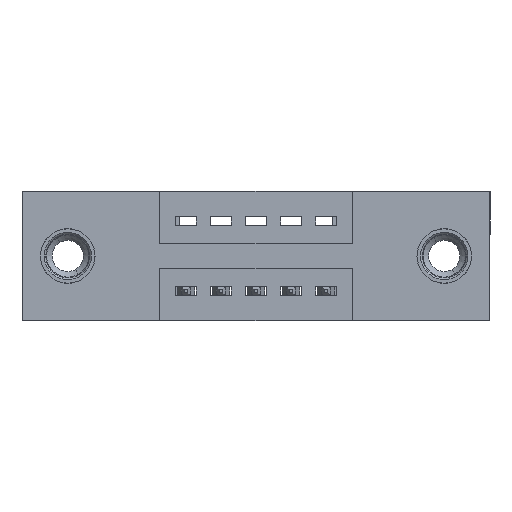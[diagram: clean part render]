
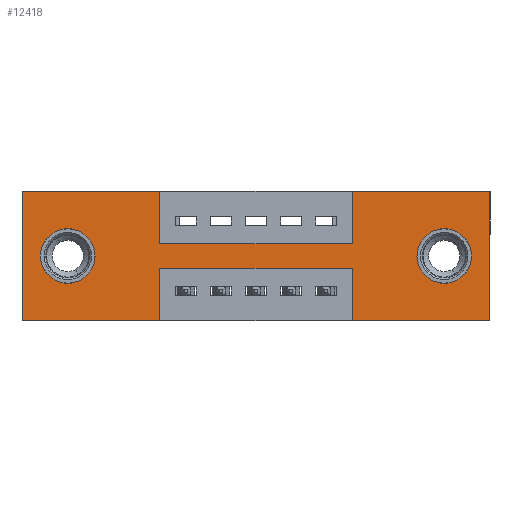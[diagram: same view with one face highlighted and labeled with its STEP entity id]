
A CAD part, front view. The second image highlights one B-rep face of the part: STEP entity #12418.
In plain terms, the highlighted planar face has unit normal (0, -1, 0).
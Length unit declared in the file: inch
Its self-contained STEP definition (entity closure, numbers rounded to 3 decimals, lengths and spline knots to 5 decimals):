
#65 = VERTEX_POINT ( 'NONE', #7563 ) ;
#151 = ORIENTED_EDGE ( 'NONE', *, *, #4716, .T. ) ;
#329 = DIRECTION ( 'NONE',  ( 0., 0., -1. ) ) ;
#368 = CARTESIAN_POINT ( 'NONE',  ( 0.13, 0., -0.263 ) ) ;
#464 = VECTOR ( 'NONE', #4039, 39.37008 ) ;
#468 = CARTESIAN_POINT ( 'NONE',  ( 0.3925, 0., -0.15 ) ) ;
#553 = AXIS2_PLACEMENT_3D ( 'NONE', #3110, #9493, #3149 ) ;
#770 = CARTESIAN_POINT ( 'NONE',  ( 1.205, 0., -0.185 ) ) ;
#801 = EDGE_CURVE ( 'NONE', #4588, #1624, #7181, .T. ) ;
#864 = LINE ( 'NONE', #12843, #6256 ) ;
#886 = CARTESIAN_POINT ( 'NONE',  ( 0.3925, 0., -0.37 ) ) ;
#897 = CARTESIAN_POINT ( 'NONE',  ( 0., 0., 0. ) ) ;
#1058 = EDGE_CURVE ( 'NONE', #5601, #1736, #4562, .T. ) ;
#1061 = VECTOR ( 'NONE', #6084, 39.37008 ) ;
#1085 = CARTESIAN_POINT ( 'NONE',  ( 1.335, 0., -0.37 ) ) ;
#1220 = LINE ( 'NONE', #897, #1061 ) ;
#1275 = VERTEX_POINT ( 'NONE', #5550 ) ;
#1297 = EDGE_CURVE ( 'NONE', #10303, #12620, #2593, .T. ) ;
#1338 = DIRECTION ( 'NONE',  ( 0., 0., 1. ) ) ;
#1624 = VERTEX_POINT ( 'NONE', #10181 ) ;
#1698 = DIRECTION ( 'NONE',  ( 1., 0., 0. ) ) ;
#1736 = VERTEX_POINT ( 'NONE', #12914 ) ;
#1891 = CARTESIAN_POINT ( 'NONE',  ( 0.9425, 0., -0.37 ) ) ;
#1957 = DIRECTION ( 'NONE',  ( -1., 0., 0. ) ) ;
#2049 = VERTEX_POINT ( 'NONE', #1085 ) ;
#2059 = ORIENTED_EDGE ( 'NONE', *, *, #7892, .F. ) ;
#2263 = DIRECTION ( 'NONE',  ( 1., 0., 0. ) ) ;
#2427 = CARTESIAN_POINT ( 'NONE',  ( 0., 0., 0. ) ) ;
#2509 = CIRCLE ( 'NONE', #6587, 0.078 ) ;
#2593 = CIRCLE ( 'NONE', #12894, 0.078 ) ;
#2631 = AXIS2_PLACEMENT_3D ( 'NONE', #3079, #10369, #8217 ) ;
#2674 = CARTESIAN_POINT ( 'NONE',  ( 0.3925, 0., -0.15 ) ) ;
#2744 = ORIENTED_EDGE ( 'NONE', *, *, #1058, .F. ) ;
#2824 = LINE ( 'NONE', #6087, #10468 ) ;
#2973 = EDGE_CURVE ( 'NONE', #9073, #12491, #11441, .T. ) ;
#3069 = CARTESIAN_POINT ( 'NONE',  ( 0.3925, 0., 0. ) ) ;
#3079 = CARTESIAN_POINT ( 'NONE',  ( 0.13, 0., -0.185 ) ) ;
#3110 = CARTESIAN_POINT ( 'NONE',  ( 0., 0., -0.37 ) ) ;
#3149 = DIRECTION ( 'NONE',  ( 0., 0., -1. ) ) ;
#3152 = EDGE_LOOP ( 'NONE', ( #11477, #5903 ) ) ;
#3196 = PLANE ( 'NONE',  #553 ) ;
#3593 = VERTEX_POINT ( 'NONE', #12208 ) ;
#3740 = CARTESIAN_POINT ( 'NONE',  ( 1.205, 0., -0.185 ) ) ;
#4039 = DIRECTION ( 'NONE',  ( -1., 0., 0. ) ) ;
#4060 = VECTOR ( 'NONE', #1338, 39.37008 ) ;
#4089 = ORIENTED_EDGE ( 'NONE', *, *, #2973, .F. ) ;
#4096 = VECTOR ( 'NONE', #6308, 39.37008 ) ;
#4217 = CARTESIAN_POINT ( 'NONE',  ( 0.3925, 0., 0. ) ) ;
#4244 = ORIENTED_EDGE ( 'NONE', *, *, #5753, .F. ) ;
#4419 = CARTESIAN_POINT ( 'NONE',  ( 0.3925, 0., -0.22 ) ) ;
#4469 = DIRECTION ( 'NONE',  ( -1., 0., 0. ) ) ;
#4562 = LINE ( 'NONE', #11212, #464 ) ;
#4588 = VERTEX_POINT ( 'NONE', #468 ) ;
#4716 = EDGE_CURVE ( 'NONE', #12620, #10303, #12542, .T. ) ;
#4994 = VECTOR ( 'NONE', #1957, 39.37008 ) ;
#5079 = VERTEX_POINT ( 'NONE', #5829 ) ;
#5218 = CARTESIAN_POINT ( 'NONE',  ( 0.9425, 0., -0.22 ) ) ;
#5248 = CARTESIAN_POINT ( 'NONE',  ( 0.13, 0., -0.107 ) ) ;
#5309 = CARTESIAN_POINT ( 'NONE',  ( 0.9425, 0., -0.37 ) ) ;
#5371 = FACE_OUTER_BOUND ( 'NONE', #10951, .T. ) ;
#5502 = LINE ( 'NONE', #2427, #4060 ) ;
#5550 = CARTESIAN_POINT ( 'NONE',  ( 1.205, 0., -0.107 ) ) ;
#5601 = VERTEX_POINT ( 'NONE', #886 ) ;
#5628 = DIRECTION ( 'NONE',  ( 0., 0., -1. ) ) ;
#5699 = DIRECTION ( 'NONE',  ( 0., 1., 0. ) ) ;
#5753 = EDGE_CURVE ( 'NONE', #1736, #9073, #5502, .T. ) ;
#5829 = CARTESIAN_POINT ( 'NONE',  ( 1.205, 0., -0.263 ) ) ;
#5903 = ORIENTED_EDGE ( 'NONE', *, *, #12830, .T. ) ;
#5971 = ORIENTED_EDGE ( 'NONE', *, *, #6689, .F. ) ;
#6015 = DIRECTION ( 'NONE',  ( 0., 0., -1. ) ) ;
#6084 = DIRECTION ( 'NONE',  ( 1., 0., 0. ) ) ;
#6087 = CARTESIAN_POINT ( 'NONE',  ( 0.9425, 0., 0. ) ) ;
#6156 = ORIENTED_EDGE ( 'NONE', *, *, #10649, .F. ) ;
#6213 = DIRECTION ( 'NONE',  ( 0., 0., 1. ) ) ;
#6256 = VECTOR ( 'NONE', #329, 39.37008 ) ;
#6308 = DIRECTION ( 'NONE',  ( 0., 0., -1. ) ) ;
#6344 = VECTOR ( 'NONE', #1698, 39.37008 ) ;
#6358 = LINE ( 'NONE', #3069, #4096 ) ;
#6478 = CARTESIAN_POINT ( 'NONE',  ( 0., 0., 0. ) ) ;
#6587 = AXIS2_PLACEMENT_3D ( 'NONE', #3740, #5699, #13011 ) ;
#6689 = EDGE_CURVE ( 'NONE', #11831, #3593, #8756, .T. ) ;
#6759 = EDGE_CURVE ( 'NONE', #3593, #5601, #10844, .T. ) ;
#7181 = LINE ( 'NONE', #2674, #6344 ) ;
#7563 = CARTESIAN_POINT ( 'NONE',  ( 0.9425, 0., 0. ) ) ;
#7619 = VECTOR ( 'NONE', #4469, 39.37008 ) ;
#7713 = CARTESIAN_POINT ( 'NONE',  ( 0.3925, 0., -0.37 ) ) ;
#7892 = EDGE_CURVE ( 'NONE', #8366, #2049, #864, .T. ) ;
#7946 = EDGE_CURVE ( 'NONE', #1275, #5079, #2509, .T. ) ;
#8115 = EDGE_LOOP ( 'NONE', ( #11945, #151 ) ) ;
#8217 = DIRECTION ( 'NONE',  ( 0., 0., 1. ) ) ;
#8252 = EDGE_CURVE ( 'NONE', #13264, #11831, #10004, .T. ) ;
#8327 = VECTOR ( 'NONE', #2263, 39.37008 ) ;
#8366 = VERTEX_POINT ( 'NONE', #9473 ) ;
#8664 = FACE_BOUND ( 'NONE', #8115, .T. ) ;
#8756 = LINE ( 'NONE', #4419, #7619 ) ;
#9070 = DIRECTION ( 'NONE',  ( 0., 0., 1. ) ) ;
#9073 = VERTEX_POINT ( 'NONE', #10957 ) ;
#9200 = EDGE_CURVE ( 'NONE', #65, #8366, #1220, .T. ) ;
#9285 = EDGE_CURVE ( 'NONE', #2049, #13264, #12331, .T. ) ;
#9306 = ORIENTED_EDGE ( 'NONE', *, *, #9285, .F. ) ;
#9473 = CARTESIAN_POINT ( 'NONE',  ( 1.335, 0., 0. ) ) ;
#9493 = DIRECTION ( 'NONE',  ( 0., -1., 0. ) ) ;
#9907 = AXIS2_PLACEMENT_3D ( 'NONE', #770, #12274, #6015 ) ;
#10004 = LINE ( 'NONE', #5309, #10316 ) ;
#10155 = ORIENTED_EDGE ( 'NONE', *, *, #801, .F. ) ;
#10181 = CARTESIAN_POINT ( 'NONE',  ( 0.9425, 0., -0.15 ) ) ;
#10303 = VERTEX_POINT ( 'NONE', #5248 ) ;
#10316 = VECTOR ( 'NONE', #6213, 39.37008 ) ;
#10369 = DIRECTION ( 'NONE',  ( 0., 1., 0. ) ) ;
#10468 = VECTOR ( 'NONE', #9070, 39.37008 ) ;
#10506 = ORIENTED_EDGE ( 'NONE', *, *, #11844, .F. ) ;
#10649 = EDGE_CURVE ( 'NONE', #1624, #65, #2824, .T. ) ;
#10675 = VECTOR ( 'NONE', #5628, 39.37008 ) ;
#10844 = LINE ( 'NONE', #7713, #10675 ) ;
#10849 = ORIENTED_EDGE ( 'NONE', *, *, #9200, .F. ) ;
#10951 = EDGE_LOOP ( 'NONE', ( #12012, #5971, #13462, #9306, #2059, #10849, #6156, #10155, #10506, #4089, #4244, #2744 ) ) ;
#10957 = CARTESIAN_POINT ( 'NONE',  ( 0., 0., 0. ) ) ;
#11212 = CARTESIAN_POINT ( 'NONE',  ( 0., 0., -0.37 ) ) ;
#11397 = CIRCLE ( 'NONE', #9907, 0.078 ) ;
#11441 = LINE ( 'NONE', #6478, #8327 ) ;
#11477 = ORIENTED_EDGE ( 'NONE', *, *, #7946, .T. ) ;
#11671 = DIRECTION ( 'NONE',  ( 0., 1., 0. ) ) ;
#11831 = VERTEX_POINT ( 'NONE', #5218 ) ;
#11844 = EDGE_CURVE ( 'NONE', #12491, #4588, #6358, .T. ) ;
#11908 = FACE_BOUND ( 'NONE', #3152, .T. ) ;
#11945 = ORIENTED_EDGE ( 'NONE', *, *, #1297, .T. ) ;
#12012 = ORIENTED_EDGE ( 'NONE', *, *, #6759, .F. ) ;
#12208 = CARTESIAN_POINT ( 'NONE',  ( 0.3925, 0., -0.22 ) ) ;
#12274 = DIRECTION ( 'NONE',  ( 0., 1., 0. ) ) ;
#12331 = LINE ( 'NONE', #12469, #4994 ) ;
#12418 = ADVANCED_FACE ( 'NONE', ( #11908, #8664, #5371 ), #3196, .T. ) ;
#12469 = CARTESIAN_POINT ( 'NONE',  ( 0., 0., -0.37 ) ) ;
#12491 = VERTEX_POINT ( 'NONE', #4217 ) ;
#12542 = CIRCLE ( 'NONE', #2631, 0.078 ) ;
#12620 = VERTEX_POINT ( 'NONE', #368 ) ;
#12722 = DIRECTION ( 'NONE',  ( 0., 0., 1. ) ) ;
#12830 = EDGE_CURVE ( 'NONE', #5079, #1275, #11397, .T. ) ;
#12843 = CARTESIAN_POINT ( 'NONE',  ( 1.335, 0., 0. ) ) ;
#12856 = CARTESIAN_POINT ( 'NONE',  ( 0.13, 0., -0.185 ) ) ;
#12894 = AXIS2_PLACEMENT_3D ( 'NONE', #12856, #11671, #12722 ) ;
#12914 = CARTESIAN_POINT ( 'NONE',  ( 0., 0., -0.37 ) ) ;
#13011 = DIRECTION ( 'NONE',  ( 0., 0., -1. ) ) ;
#13264 = VERTEX_POINT ( 'NONE', #1891 ) ;
#13462 = ORIENTED_EDGE ( 'NONE', *, *, #8252, .F. ) ;
